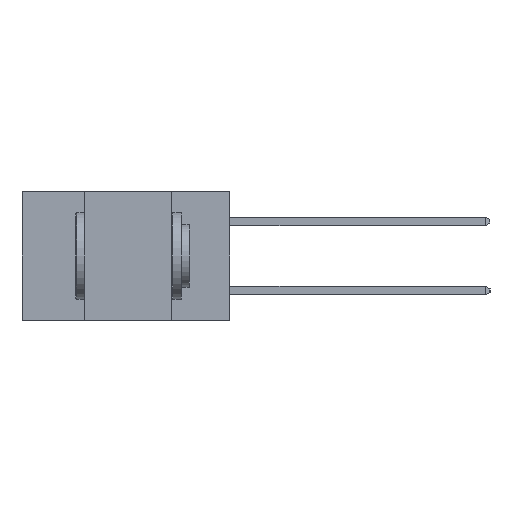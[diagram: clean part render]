
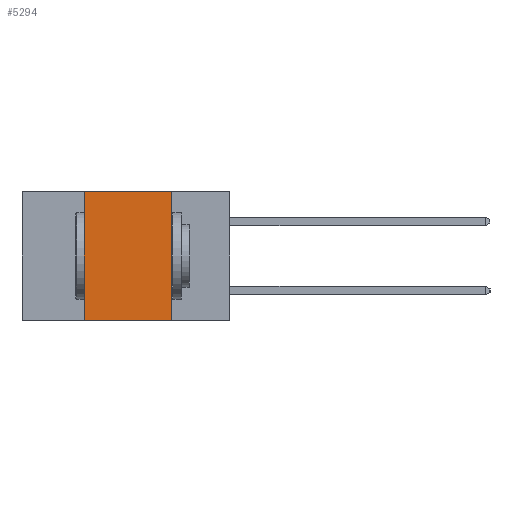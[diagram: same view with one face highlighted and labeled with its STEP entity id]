
A CAD part, left-side view. The second image highlights one B-rep face of the part: STEP entity #5294.
In plain terms, the highlighted planar face has unit normal (-1, 0, 0).
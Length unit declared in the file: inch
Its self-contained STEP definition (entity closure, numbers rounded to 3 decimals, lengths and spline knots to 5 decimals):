
#144 = AXIS2_PLACEMENT_3D ( 'NONE', #11177, #11074, #10970 ) ;
#732 = DIRECTION ( 'NONE',  ( 0., 0., -1. ) ) ;
#762 = CARTESIAN_POINT ( 'NONE',  ( 0., 0.17, -0.37 ) ) ;
#2134 = LINE ( 'NONE', #762, #14447 ) ;
#2214 = DIRECTION ( 'NONE',  ( 0., -1., 0. ) ) ;
#2254 = CARTESIAN_POINT ( 'NONE',  ( 0., 0.6, -0.37 ) ) ;
#2419 = LINE ( 'NONE', #2254, #14376 ) ;
#2574 = CARTESIAN_POINT ( 'NONE',  ( 0., 0.42, 0. ) ) ;
#2639 = VERTEX_POINT ( 'NONE', #8724 ) ;
#3767 = DIRECTION ( 'NONE',  ( 0., -1., 0. ) ) ;
#3901 = CARTESIAN_POINT ( 'NONE',  ( 0., 0.6, 0. ) ) ;
#3937 = VERTEX_POINT ( 'NONE', #7660 ) ;
#4669 = EDGE_CURVE ( 'NONE', #12765, #3937, #2134, .T. ) ;
#5040 = LINE ( 'NONE', #13508, #8343 ) ;
#5074 = EDGE_LOOP ( 'NONE', ( #10152, #6925, #15089, #14764 ) ) ;
#5281 = CARTESIAN_POINT ( 'NONE',  ( 0., 0.17, 0. ) ) ;
#5294 = ADVANCED_FACE ( 'NONE', ( #12324 ), #11659, .F. ) ;
#6925 = ORIENTED_EDGE ( 'NONE', *, *, #8183, .F. ) ;
#7472 = EDGE_CURVE ( 'NONE', #2639, #3937, #2419, .T. ) ;
#7660 = CARTESIAN_POINT ( 'NONE',  ( 0., 0.17, -0.37 ) ) ;
#7966 = VECTOR ( 'NONE', #3767, 39.37008 ) ;
#8183 = EDGE_CURVE ( 'NONE', #12952, #12765, #11155, .T. ) ;
#8343 = VECTOR ( 'NONE', #13586, 39.37008 ) ;
#8724 = CARTESIAN_POINT ( 'NONE',  ( 0., 0.42, -0.37 ) ) ;
#10101 = EDGE_CURVE ( 'NONE', #2639, #12952, #5040, .T. ) ;
#10152 = ORIENTED_EDGE ( 'NONE', *, *, #4669, .F. ) ;
#10970 = DIRECTION ( 'NONE',  ( 0., 0., -1. ) ) ;
#11074 = DIRECTION ( 'NONE',  ( 1., 0., 0. ) ) ;
#11155 = LINE ( 'NONE', #3901, #7966 ) ;
#11177 = CARTESIAN_POINT ( 'NONE',  ( 0., 0.6, 0. ) ) ;
#11659 = PLANE ( 'NONE',  #144 ) ;
#12324 = FACE_OUTER_BOUND ( 'NONE', #5074, .T. ) ;
#12765 = VERTEX_POINT ( 'NONE', #5281 ) ;
#12952 = VERTEX_POINT ( 'NONE', #2574 ) ;
#13508 = CARTESIAN_POINT ( 'NONE',  ( 0., 0.42, -0.37 ) ) ;
#13586 = DIRECTION ( 'NONE',  ( 0., 0., 1. ) ) ;
#14376 = VECTOR ( 'NONE', #2214, 39.37008 ) ;
#14447 = VECTOR ( 'NONE', #732, 39.37008 ) ;
#14764 = ORIENTED_EDGE ( 'NONE', *, *, #7472, .T. ) ;
#15089 = ORIENTED_EDGE ( 'NONE', *, *, #10101, .F. ) ;
